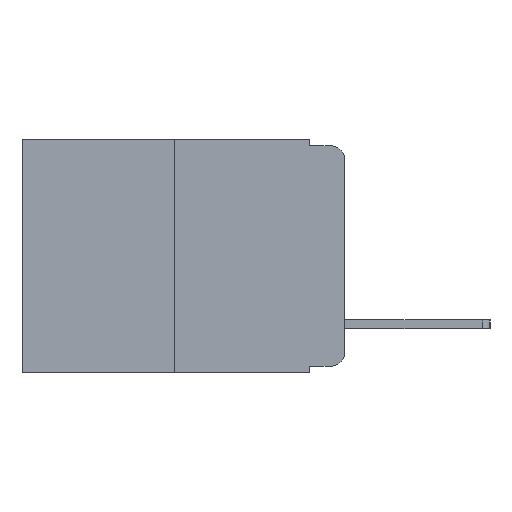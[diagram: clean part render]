
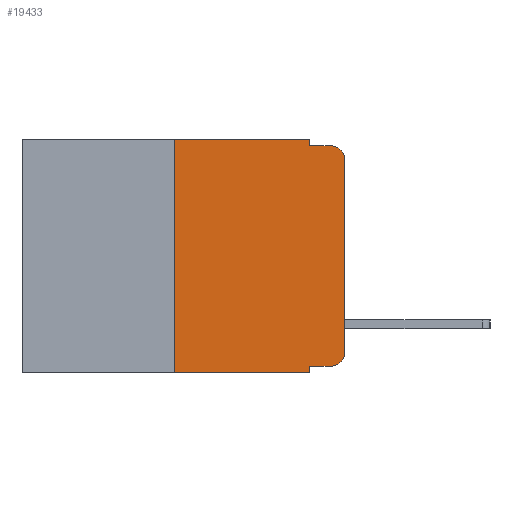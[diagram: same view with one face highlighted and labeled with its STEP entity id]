
A CAD part, left-side view. The second image highlights one B-rep face of the part: STEP entity #19433.
In plain terms, the highlighted planar face has unit normal (-1, 0, 0).
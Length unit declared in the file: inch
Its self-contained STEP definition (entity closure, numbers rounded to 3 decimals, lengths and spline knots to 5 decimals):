
#37 = ORIENTED_EDGE ( 'NONE', *, *, #4912, .F. ) ;
#179 = LINE ( 'NONE', #2550, #22682 ) ;
#346 = VECTOR ( 'NONE', #16622, 39.37008 ) ;
#1166 = AXIS2_PLACEMENT_3D ( 'NONE', #12462, #17675, #7174 ) ;
#1587 = VERTEX_POINT ( 'NONE', #19166 ) ;
#1783 = ORIENTED_EDGE ( 'NONE', *, *, #3091, .T. ) ;
#1789 = DIRECTION ( 'NONE',  ( 0., 0., 1. ) ) ;
#2136 = EDGE_CURVE ( 'NONE', #21459, #17389, #14687, .T. ) ;
#2500 = VERTEX_POINT ( 'NONE', #20428 ) ;
#2550 = CARTESIAN_POINT ( 'NONE',  ( 0., 0., 0. ) ) ;
#2583 = LINE ( 'NONE', #12530, #6259 ) ;
#2904 = CARTESIAN_POINT ( 'NONE',  ( 0., 0.473, -0.343 ) ) ;
#3091 = EDGE_CURVE ( 'NONE', #6408, #2500, #5184, .T. ) ;
#3382 = LINE ( 'NONE', #18149, #16935 ) ;
#3754 = VECTOR ( 'NONE', #15449, 39.37008 ) ;
#4045 = DIRECTION ( 'NONE',  ( 0., 0., -1. ) ) ;
#4890 = LINE ( 'NONE', #15855, #3754 ) ;
#4912 = EDGE_CURVE ( 'NONE', #22414, #1587, #16513, .T. ) ;
#5184 = CIRCLE ( 'NONE', #16570, 0.02 ) ;
#5425 = DIRECTION ( 'NONE',  ( 0., 0., -1. ) ) ;
#5479 = ORIENTED_EDGE ( 'NONE', *, *, #2136, .T. ) ;
#5487 = EDGE_CURVE ( 'NONE', #8917, #6408, #4890, .T. ) ;
#6104 = VECTOR ( 'NONE', #15422, 39.37008 ) ;
#6259 = VECTOR ( 'NONE', #5425, 39.37008 ) ;
#6408 = VERTEX_POINT ( 'NONE', #11768 ) ;
#6701 = EDGE_CURVE ( 'NONE', #8917, #17389, #2583, .T. ) ;
#7174 = DIRECTION ( 'NONE',  ( 0., 0., -1. ) ) ;
#7460 = ORIENTED_EDGE ( 'NONE', *, *, #13845, .T. ) ;
#7662 = CARTESIAN_POINT ( 'NONE',  ( 0., 0.051, -0.343 ) ) ;
#7910 = EDGE_CURVE ( 'NONE', #21459, #22414, #18308, .T. ) ;
#8006 = DIRECTION ( 'NONE',  ( 0., 0., 1. ) ) ;
#8597 = ORIENTED_EDGE ( 'NONE', *, *, #11479, .F. ) ;
#8887 = PLANE ( 'NONE',  #1166 ) ;
#8917 = VERTEX_POINT ( 'NONE', #22318 ) ;
#9130 = ORIENTED_EDGE ( 'NONE', *, *, #10278, .F. ) ;
#9177 = CARTESIAN_POINT ( 'NONE',  ( 0., 0., -0.03 ) ) ;
#9649 = VERTEX_POINT ( 'NONE', #11098 ) ;
#10278 = EDGE_CURVE ( 'NONE', #1587, #15394, #3382, .T. ) ;
#10414 = CARTESIAN_POINT ( 'NONE',  ( 0., 0.02, -0.03 ) ) ;
#10531 = CIRCLE ( 'NONE', #17013, 0.02 ) ;
#11098 = CARTESIAN_POINT ( 'NONE',  ( 0., 0.02, -0.01 ) ) ;
#11332 = VECTOR ( 'NONE', #17459, 39.37008 ) ;
#11479 = EDGE_CURVE ( 'NONE', #15394, #9649, #16059, .T. ) ;
#11768 = CARTESIAN_POINT ( 'NONE',  ( 0., 0.02, -0.333 ) ) ;
#11910 = CARTESIAN_POINT ( 'NONE',  ( 0., 0.051, -0.01 ) ) ;
#12211 = DIRECTION ( 'NONE',  ( 0., 0., -1. ) ) ;
#12405 = VERTEX_POINT ( 'NONE', #9177 ) ;
#12462 = CARTESIAN_POINT ( 'NONE',  ( 0., 0.473, 0. ) ) ;
#12530 = CARTESIAN_POINT ( 'NONE',  ( 0., 0.051, 0. ) ) ;
#12677 = EDGE_CURVE ( 'NONE', #12405, #9649, #10531, .T. ) ;
#13170 = VECTOR ( 'NONE', #1789, 39.37008 ) ;
#13606 = EDGE_LOOP ( 'NONE', ( #7460, #17349, #8597, #9130, #37, #18981, #5479, #14934, #15465, #1783 ) ) ;
#13845 = EDGE_CURVE ( 'NONE', #2500, #12405, #179, .T. ) ;
#14541 = CARTESIAN_POINT ( 'NONE',  ( 0., 0.02, -0.313 ) ) ;
#14687 = LINE ( 'NONE', #2904, #346 ) ;
#14774 = FACE_OUTER_BOUND ( 'NONE', #13606, .T. ) ;
#14934 = ORIENTED_EDGE ( 'NONE', *, *, #6701, .F. ) ;
#14964 = CARTESIAN_POINT ( 'NONE',  ( 0., 0.25, -0.343 ) ) ;
#15394 = VERTEX_POINT ( 'NONE', #18789 ) ;
#15422 = DIRECTION ( 'NONE',  ( 0., -1., 0. ) ) ;
#15449 = DIRECTION ( 'NONE',  ( 0., -1., 0. ) ) ;
#15465 = ORIENTED_EDGE ( 'NONE', *, *, #5487, .T. ) ;
#15855 = CARTESIAN_POINT ( 'NONE',  ( 0., 0.051, -0.333 ) ) ;
#16059 = LINE ( 'NONE', #11910, #6104 ) ;
#16170 = CARTESIAN_POINT ( 'NONE',  ( 0., 0.473, 0. ) ) ;
#16513 = LINE ( 'NONE', #16170, #11332 ) ;
#16570 = AXIS2_PLACEMENT_3D ( 'NONE', #14541, #19148, #17631 ) ;
#16622 = DIRECTION ( 'NONE',  ( 0., -1., 0. ) ) ;
#16935 = VECTOR ( 'NONE', #4045, 39.37008 ) ;
#17013 = AXIS2_PLACEMENT_3D ( 'NONE', #10414, #22636, #12211 ) ;
#17349 = ORIENTED_EDGE ( 'NONE', *, *, #12677, .T. ) ;
#17389 = VERTEX_POINT ( 'NONE', #7662 ) ;
#17459 = DIRECTION ( 'NONE',  ( 0., -1., 0. ) ) ;
#17631 = DIRECTION ( 'NONE',  ( 0., 0., -1. ) ) ;
#17675 = DIRECTION ( 'NONE',  ( 1., 0., 0. ) ) ;
#18149 = CARTESIAN_POINT ( 'NONE',  ( 0., 0.051, 0. ) ) ;
#18308 = LINE ( 'NONE', #22977, #13170 ) ;
#18789 = CARTESIAN_POINT ( 'NONE',  ( 0., 0.051, -0.01 ) ) ;
#18981 = ORIENTED_EDGE ( 'NONE', *, *, #7910, .F. ) ;
#19148 = DIRECTION ( 'NONE',  ( -1., 0., 0. ) ) ;
#19166 = CARTESIAN_POINT ( 'NONE',  ( 0., 0.051, 0. ) ) ;
#19433 = ADVANCED_FACE ( 'NONE', ( #14774 ), #8887, .F. ) ;
#20386 = CARTESIAN_POINT ( 'NONE',  ( 0., 0.25, 0. ) ) ;
#20428 = CARTESIAN_POINT ( 'NONE',  ( 0., 0., -0.313 ) ) ;
#21459 = VERTEX_POINT ( 'NONE', #14964 ) ;
#22318 = CARTESIAN_POINT ( 'NONE',  ( 0., 0.051, -0.333 ) ) ;
#22414 = VERTEX_POINT ( 'NONE', #20386 ) ;
#22636 = DIRECTION ( 'NONE',  ( -1., 0., 0. ) ) ;
#22682 = VECTOR ( 'NONE', #8006, 39.37008 ) ;
#22977 = CARTESIAN_POINT ( 'NONE',  ( 0., 0.25, 0. ) ) ;
